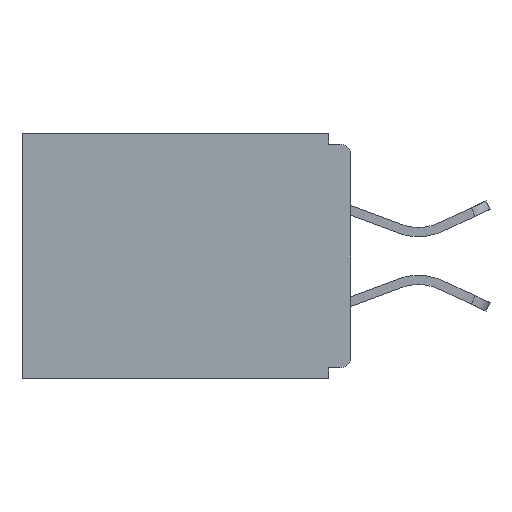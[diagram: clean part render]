
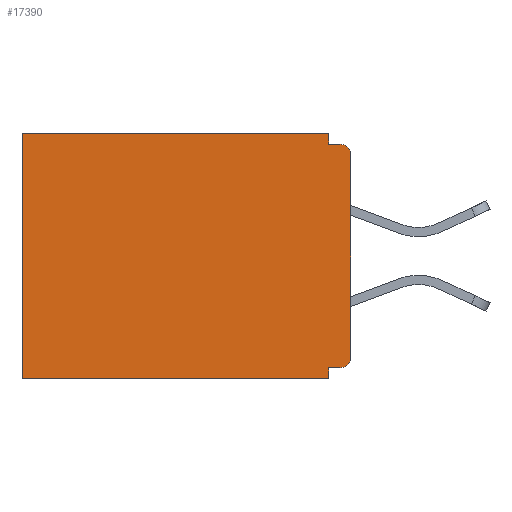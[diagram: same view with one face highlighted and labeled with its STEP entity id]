
A CAD part, left-side view. The second image highlights one B-rep face of the part: STEP entity #17390.
In plain terms, the highlighted planar face has unit normal (-1, 0, 0).
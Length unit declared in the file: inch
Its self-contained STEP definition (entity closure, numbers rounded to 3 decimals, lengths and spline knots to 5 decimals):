
#117 = CARTESIAN_POINT ( 'NONE',  ( 0.298, 0., -0.03 ) ) ;
#146 = ORIENTED_EDGE ( 'NONE', *, *, #15350, .T. ) ;
#302 = VERTEX_POINT ( 'NONE', #8108 ) ;
#334 = VERTEX_POINT ( 'NONE', #9832 ) ;
#434 = ORIENTED_EDGE ( 'NONE', *, *, #18889, .T. ) ;
#673 = VERTEX_POINT ( 'NONE', #13465 ) ;
#1137 = PLANE ( 'NONE',  #18765 ) ;
#1501 = EDGE_CURVE ( 'NONE', #12187, #18998, #3808, .T. ) ;
#1818 = VERTEX_POINT ( 'NONE', #16975 ) ;
#2009 = LINE ( 'NONE', #17903, #13740 ) ;
#2461 = ORIENTED_EDGE ( 'NONE', *, *, #13133, .F. ) ;
#2692 = DIRECTION ( 'NONE',  ( 1., 0., 0. ) ) ;
#2777 = AXIS2_PLACEMENT_3D ( 'NONE', #5376, #9951, #8492 ) ;
#2832 = CARTESIAN_POINT ( 'NONE',  ( 0.298, 0.015, -0.03 ) ) ;
#2842 = CARTESIAN_POINT ( 'NONE',  ( 0.298, 0.46, -0.343 ) ) ;
#3045 = VECTOR ( 'NONE', #10818, 39.37008 ) ;
#3176 = CARTESIAN_POINT ( 'NONE',  ( 0.298, 0.015, -0.015 ) ) ;
#3294 = LINE ( 'NONE', #14755, #6101 ) ;
#3345 = VECTOR ( 'NONE', #3851, 39.37008 ) ;
#3500 = EDGE_CURVE ( 'NONE', #1818, #11500, #9897, .T. ) ;
#3788 = CARTESIAN_POINT ( 'NONE',  ( 0.298, 0.031, -0.343 ) ) ;
#3808 = LINE ( 'NONE', #8553, #3345 ) ;
#3851 = DIRECTION ( 'NONE',  ( 0., 0., -1. ) ) ;
#4153 = VERTEX_POINT ( 'NONE', #6669 ) ;
#4472 = ORIENTED_EDGE ( 'NONE', *, *, #1501, .F. ) ;
#4898 = EDGE_LOOP ( 'NONE', ( #19419, #18975, #13810, #146, #434, #6535, #17160, #2461, #8455, #4472 ) ) ;
#5376 = CARTESIAN_POINT ( 'NONE',  ( 0.298, 0.015, -0.313 ) ) ;
#5675 = DIRECTION ( 'NONE',  ( 0., 1., 0. ) ) ;
#6056 = CARTESIAN_POINT ( 'NONE',  ( 0.298, 0., -0.328 ) ) ;
#6064 = VECTOR ( 'NONE', #5675, 39.37008 ) ;
#6101 = VECTOR ( 'NONE', #19160, 39.37008 ) ;
#6535 = ORIENTED_EDGE ( 'NONE', *, *, #18297, .F. ) ;
#6669 = CARTESIAN_POINT ( 'NONE',  ( 0.298, 0.031, 0. ) ) ;
#7109 = DIRECTION ( 'NONE',  ( 0., 0., -1. ) ) ;
#7156 = LINE ( 'NONE', #9693, #12324 ) ;
#7580 = VECTOR ( 'NONE', #10422, 39.37008 ) ;
#7727 = LINE ( 'NONE', #3788, #7960 ) ;
#7770 = CARTESIAN_POINT ( 'NONE',  ( 0.298, 0., -0.015 ) ) ;
#7960 = VECTOR ( 'NONE', #9946, 39.37008 ) ;
#8108 = CARTESIAN_POINT ( 'NONE',  ( 0.298, 0.031, -0.343 ) ) ;
#8186 = EDGE_CURVE ( 'NONE', #16256, #18998, #14728, .T. ) ;
#8455 = ORIENTED_EDGE ( 'NONE', *, *, #8186, .T. ) ;
#8492 = DIRECTION ( 'NONE',  ( 0., 0., -1. ) ) ;
#8553 = CARTESIAN_POINT ( 'NONE',  ( 0.298, 0., 0. ) ) ;
#8909 = EDGE_CURVE ( 'NONE', #673, #302, #2009, .T. ) ;
#9591 = CARTESIAN_POINT ( 'NONE',  ( 0.298, 0., -0.313 ) ) ;
#9693 = CARTESIAN_POINT ( 'NONE',  ( 0.298, 0., -0.343 ) ) ;
#9832 = CARTESIAN_POINT ( 'NONE',  ( 0.298, 0.46, 0. ) ) ;
#9897 = LINE ( 'NONE', #7770, #3045 ) ;
#9946 = DIRECTION ( 'NONE',  ( 0., 0., -1. ) ) ;
#9951 = DIRECTION ( 'NONE',  ( -1., 0., 0. ) ) ;
#10396 = DIRECTION ( 'NONE',  ( 0., 0., -1. ) ) ;
#10422 = DIRECTION ( 'NONE',  ( 0., 1., 0. ) ) ;
#10818 = DIRECTION ( 'NONE',  ( 0., -1., 0. ) ) ;
#11168 = CARTESIAN_POINT ( 'NONE',  ( 0.298, 0.015, -0.328 ) ) ;
#11500 = VERTEX_POINT ( 'NONE', #3176 ) ;
#12187 = VERTEX_POINT ( 'NONE', #117 ) ;
#12324 = VECTOR ( 'NONE', #12971, 39.37008 ) ;
#12534 = LINE ( 'NONE', #6056, #7580 ) ;
#12971 = DIRECTION ( 'NONE',  ( 0., 1., 0. ) ) ;
#13131 = LINE ( 'NONE', #17383, #6064 ) ;
#13133 = EDGE_CURVE ( 'NONE', #16256, #673, #12534, .T. ) ;
#13282 = CARTESIAN_POINT ( 'NONE',  ( 0.298, 0., 0. ) ) ;
#13465 = CARTESIAN_POINT ( 'NONE',  ( 0.298, 0.031, -0.328 ) ) ;
#13740 = VECTOR ( 'NONE', #16278, 39.37008 ) ;
#13760 = FACE_OUTER_BOUND ( 'NONE', #4898, .T. ) ;
#13810 = ORIENTED_EDGE ( 'NONE', *, *, #14885, .F. ) ;
#14463 = CIRCLE ( 'NONE', #17990, 0.015 ) ;
#14728 = CIRCLE ( 'NONE', #2777, 0.015 ) ;
#14755 = CARTESIAN_POINT ( 'NONE',  ( 0.298, 0.46, 0. ) ) ;
#14847 = DIRECTION ( 'NONE',  ( -1., 0., 0. ) ) ;
#14885 = EDGE_CURVE ( 'NONE', #4153, #1818, #7727, .T. ) ;
#15350 = EDGE_CURVE ( 'NONE', #4153, #334, #13131, .T. ) ;
#16256 = VERTEX_POINT ( 'NONE', #11168 ) ;
#16278 = DIRECTION ( 'NONE',  ( 0., 0., -1. ) ) ;
#16975 = CARTESIAN_POINT ( 'NONE',  ( 0.298, 0.031, -0.015 ) ) ;
#17160 = ORIENTED_EDGE ( 'NONE', *, *, #8909, .F. ) ;
#17383 = CARTESIAN_POINT ( 'NONE',  ( 0.298, 0., 0. ) ) ;
#17390 = ADVANCED_FACE ( 'NONE', ( #13760 ), #1137, .F. ) ;
#17529 = EDGE_CURVE ( 'NONE', #12187, #11500, #14463, .T. ) ;
#17903 = CARTESIAN_POINT ( 'NONE',  ( 0.298, 0.031, -0.343 ) ) ;
#17990 = AXIS2_PLACEMENT_3D ( 'NONE', #2832, #14847, #10396 ) ;
#18297 = EDGE_CURVE ( 'NONE', #302, #18733, #7156, .T. ) ;
#18733 = VERTEX_POINT ( 'NONE', #2842 ) ;
#18765 = AXIS2_PLACEMENT_3D ( 'NONE', #13282, #2692, #7109 ) ;
#18889 = EDGE_CURVE ( 'NONE', #334, #18733, #3294, .T. ) ;
#18975 = ORIENTED_EDGE ( 'NONE', *, *, #3500, .F. ) ;
#18998 = VERTEX_POINT ( 'NONE', #9591 ) ;
#19160 = DIRECTION ( 'NONE',  ( 0., 0., -1. ) ) ;
#19419 = ORIENTED_EDGE ( 'NONE', *, *, #17529, .T. ) ;
